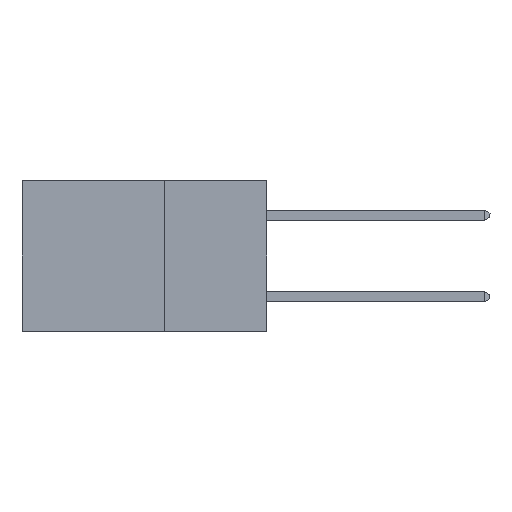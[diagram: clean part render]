
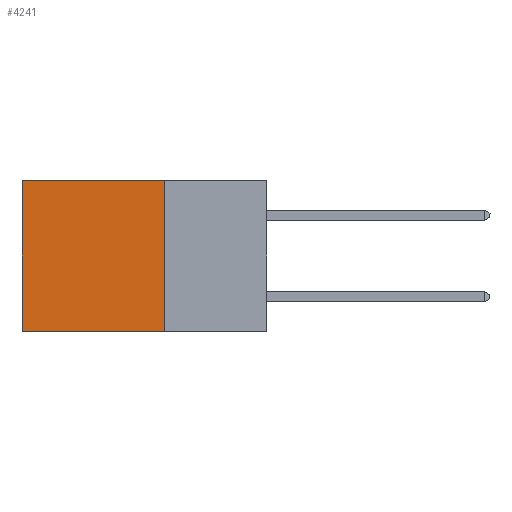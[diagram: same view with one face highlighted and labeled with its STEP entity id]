
A CAD part, left-side view. The second image highlights one B-rep face of the part: STEP entity #4241.
In plain terms, the highlighted planar face has unit normal (-1, 0, 0).
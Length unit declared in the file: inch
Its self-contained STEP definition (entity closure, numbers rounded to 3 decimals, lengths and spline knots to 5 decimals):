
#519 = LINE ( 'NONE', #859, #23604 ) ;
#859 = CARTESIAN_POINT ( 'NONE',  ( 0.2875, 0.25, 0. ) ) ;
#1203 = VERTEX_POINT ( 'NONE', #4921 ) ;
#1249 = CARTESIAN_POINT ( 'NONE',  ( 0.2875, 0.25, -0.37 ) ) ;
#4041 = VECTOR ( 'NONE', #13420, 39.37008 ) ;
#4241 = ADVANCED_FACE ( 'NONE', ( #10629 ), #11924, .F. ) ;
#4921 = CARTESIAN_POINT ( 'NONE',  ( 0.2875, 0.6, 0. ) ) ;
#5096 = DIRECTION ( 'NONE',  ( 0., 0., -1. ) ) ;
#5756 = EDGE_CURVE ( 'NONE', #1203, #12423, #7212, .T. ) ;
#6083 = VECTOR ( 'NONE', #5096, 39.37008 ) ;
#6685 = EDGE_CURVE ( 'NONE', #22488, #13990, #23398, .T. ) ;
#7212 = LINE ( 'NONE', #10441, #6083 ) ;
#7861 = CARTESIAN_POINT ( 'NONE',  ( 0.2875, 0.6, -0.37 ) ) ;
#9928 = AXIS2_PLACEMENT_3D ( 'NONE', #15585, #21173, #10220 ) ;
#10220 = DIRECTION ( 'NONE',  ( 0., 0., -1. ) ) ;
#10441 = CARTESIAN_POINT ( 'NONE',  ( 0.2875, 0.6, 0. ) ) ;
#10629 = FACE_OUTER_BOUND ( 'NONE', #14098, .T. ) ;
#11062 = ORIENTED_EDGE ( 'NONE', *, *, #5756, .T. ) ;
#11821 = VECTOR ( 'NONE', #13689, 39.37008 ) ;
#11924 = PLANE ( 'NONE',  #9928 ) ;
#12381 = LINE ( 'NONE', #17217, #11821 ) ;
#12423 = VERTEX_POINT ( 'NONE', #7861 ) ;
#12856 = ORIENTED_EDGE ( 'NONE', *, *, #18921, .T. ) ;
#13420 = DIRECTION ( 'NONE',  ( 0., 0., -1. ) ) ;
#13525 = ORIENTED_EDGE ( 'NONE', *, *, #6685, .F. ) ;
#13567 = DIRECTION ( 'NONE',  ( 0., 1., 0. ) ) ;
#13689 = DIRECTION ( 'NONE',  ( 0., 1., 0. ) ) ;
#13990 = VERTEX_POINT ( 'NONE', #1249 ) ;
#14098 = EDGE_LOOP ( 'NONE', ( #11062, #17578, #13525, #12856 ) ) ;
#15585 = CARTESIAN_POINT ( 'NONE',  ( 0.2875, 0.25, 0. ) ) ;
#17217 = CARTESIAN_POINT ( 'NONE',  ( 0.2875, 0.25, -0.37 ) ) ;
#17578 = ORIENTED_EDGE ( 'NONE', *, *, #19686, .F. ) ;
#18900 = CARTESIAN_POINT ( 'NONE',  ( 0.2875, 0.25, 0. ) ) ;
#18921 = EDGE_CURVE ( 'NONE', #22488, #1203, #519, .T. ) ;
#19686 = EDGE_CURVE ( 'NONE', #13990, #12423, #12381, .T. ) ;
#21173 = DIRECTION ( 'NONE',  ( 1., 0., 0. ) ) ;
#22488 = VERTEX_POINT ( 'NONE', #18900 ) ;
#22550 = CARTESIAN_POINT ( 'NONE',  ( 0.2875, 0.25, 0. ) ) ;
#23398 = LINE ( 'NONE', #22550, #4041 ) ;
#23604 = VECTOR ( 'NONE', #13567, 39.37008 ) ;
